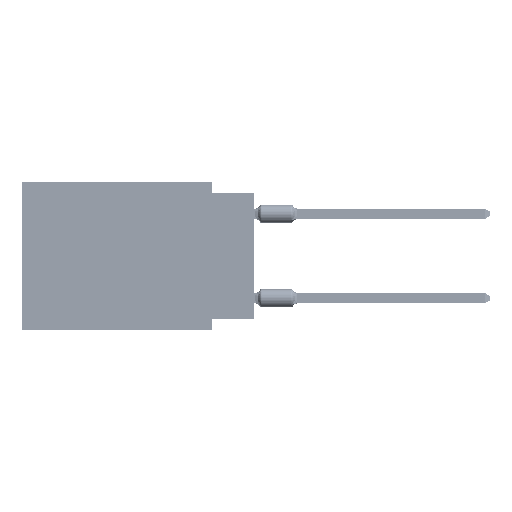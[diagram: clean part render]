
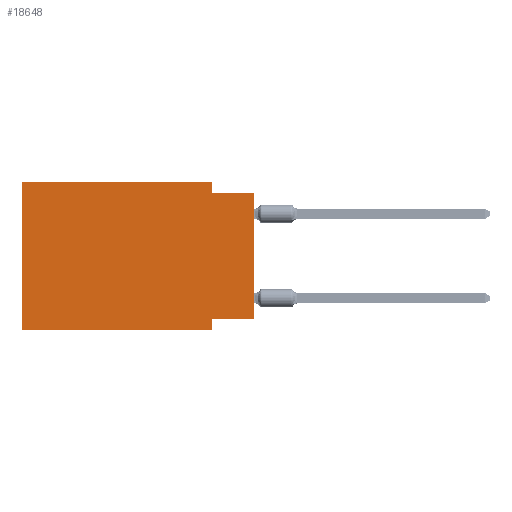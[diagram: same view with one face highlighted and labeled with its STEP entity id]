
A CAD part, left-side view. The second image highlights one B-rep face of the part: STEP entity #18648.
In plain terms, the highlighted planar face has unit normal (-1, 0, 0).
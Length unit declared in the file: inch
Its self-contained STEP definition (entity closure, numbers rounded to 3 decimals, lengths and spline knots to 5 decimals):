
#1255 = VERTEX_POINT ( 'NONE', #31636 ) ;
#1350 = EDGE_CURVE ( 'NONE', #70634, #8114, #46637, .T. ) ;
#3632 = ORIENTED_EDGE ( 'NONE', *, *, #26563, .T. ) ;
#4071 = LINE ( 'NONE', #10795, #54244 ) ;
#4739 = DIRECTION ( 'NONE',  ( 0., 0., 1. ) ) ;
#6099 = VECTOR ( 'NONE', #80054, 39.37008 ) ;
#6682 = ORIENTED_EDGE ( 'NONE', *, *, #34591, .F. ) ;
#6971 = EDGE_CURVE ( 'NONE', #55700, #53142, #4071, .T. ) ;
#7519 = EDGE_CURVE ( 'NONE', #1255, #55700, #9159, .T. ) ;
#8114 = VERTEX_POINT ( 'NONE', #39401 ) ;
#8836 = ORIENTED_EDGE ( 'NONE', *, *, #7519, .F. ) ;
#8991 = DIRECTION ( 'NONE',  ( 1., 0., 0. ) ) ;
#9159 = LINE ( 'NONE', #22427, #59217 ) ;
#9866 = DIRECTION ( 'NONE',  ( 0., 0., -1. ) ) ;
#10310 = VERTEX_POINT ( 'NONE', #69260 ) ;
#10795 = CARTESIAN_POINT ( 'NONE',  ( 0., 0., -0.025 ) ) ;
#11012 = LINE ( 'NONE', #73951, #26374 ) ;
#14127 = EDGE_CURVE ( 'NONE', #47273, #53142, #49328, .T. ) ;
#14296 = EDGE_CURVE ( 'NONE', #47273, #53185, #73774, .T. ) ;
#17582 = VECTOR ( 'NONE', #65293, 39.37008 ) ;
#18219 = CARTESIAN_POINT ( 'NONE',  ( 0., 0., 0. ) ) ;
#18648 = ADVANCED_FACE ( 'NONE', ( #41295 ), #28446, .F. ) ;
#19945 = ORIENTED_EDGE ( 'NONE', *, *, #6971, .F. ) ;
#20330 = DIRECTION ( 'NONE',  ( 0., -1., 0. ) ) ;
#21997 = CARTESIAN_POINT ( 'NONE',  ( 0., 0.55, -0.35 ) ) ;
#22427 = CARTESIAN_POINT ( 'NONE',  ( 0., 0.1, 0. ) ) ;
#24600 = EDGE_CURVE ( 'NONE', #8114, #1255, #81831, .T. ) ;
#26212 = CARTESIAN_POINT ( 'NONE',  ( 0., 0., -0.325 ) ) ;
#26374 = VECTOR ( 'NONE', #48026, 39.37008 ) ;
#26563 = EDGE_CURVE ( 'NONE', #70634, #10310, #11012, .T. ) ;
#28446 = PLANE ( 'NONE',  #42742 ) ;
#29274 = VECTOR ( 'NONE', #78388, 39.37008 ) ;
#29802 = VECTOR ( 'NONE', #20330, 39.37008 ) ;
#31636 = CARTESIAN_POINT ( 'NONE',  ( 0., 0.1, 0. ) ) ;
#32499 = EDGE_LOOP ( 'NONE', ( #65404, #19945, #8836, #62683, #41737, #3632, #6682, #44128 ) ) ;
#34020 = VECTOR ( 'NONE', #4739, 39.37008 ) ;
#34437 = CARTESIAN_POINT ( 'NONE',  ( 0., 0.1, -0.35 ) ) ;
#34591 = EDGE_CURVE ( 'NONE', #53185, #10310, #67433, .T. ) ;
#36851 = DIRECTION ( 'NONE',  ( 0., -1., 0. ) ) ;
#39401 = CARTESIAN_POINT ( 'NONE',  ( 0., 0.55, 0. ) ) ;
#41295 = FACE_OUTER_BOUND ( 'NONE', #32499, .T. ) ;
#41737 = ORIENTED_EDGE ( 'NONE', *, *, #1350, .F. ) ;
#42742 = AXIS2_PLACEMENT_3D ( 'NONE', #80630, #8991, #54689 ) ;
#44128 = ORIENTED_EDGE ( 'NONE', *, *, #14296, .F. ) ;
#46637 = LINE ( 'NONE', #84563, #29274 ) ;
#47273 = VERTEX_POINT ( 'NONE', #76887 ) ;
#48026 = DIRECTION ( 'NONE',  ( 0., -1., 0. ) ) ;
#49328 = LINE ( 'NONE', #18219, #34020 ) ;
#53142 = VERTEX_POINT ( 'NONE', #71591 ) ;
#53185 = VERTEX_POINT ( 'NONE', #72151 ) ;
#54244 = VECTOR ( 'NONE', #36851, 39.37008 ) ;
#54689 = DIRECTION ( 'NONE',  ( 0., 0., -1. ) ) ;
#55700 = VERTEX_POINT ( 'NONE', #75959 ) ;
#59217 = VECTOR ( 'NONE', #9866, 39.37008 ) ;
#62683 = ORIENTED_EDGE ( 'NONE', *, *, #24600, .F. ) ;
#65293 = DIRECTION ( 'NONE',  ( 0., 1., 0. ) ) ;
#65404 = ORIENTED_EDGE ( 'NONE', *, *, #14127, .T. ) ;
#67433 = LINE ( 'NONE', #34437, #6099 ) ;
#69260 = CARTESIAN_POINT ( 'NONE',  ( 0., 0.1, -0.35 ) ) ;
#70634 = VERTEX_POINT ( 'NONE', #21997 ) ;
#71591 = CARTESIAN_POINT ( 'NONE',  ( 0., 0., -0.025 ) ) ;
#72151 = CARTESIAN_POINT ( 'NONE',  ( 0., 0.1, -0.325 ) ) ;
#72571 = CARTESIAN_POINT ( 'NONE',  ( 0., 0.55, 0. ) ) ;
#73774 = LINE ( 'NONE', #26212, #17582 ) ;
#73951 = CARTESIAN_POINT ( 'NONE',  ( 0., 0.55, -0.35 ) ) ;
#75959 = CARTESIAN_POINT ( 'NONE',  ( 0., 0.1, -0.025 ) ) ;
#76887 = CARTESIAN_POINT ( 'NONE',  ( 0., 0., -0.325 ) ) ;
#78388 = DIRECTION ( 'NONE',  ( 0., 0., 1. ) ) ;
#80054 = DIRECTION ( 'NONE',  ( 0., 0., -1. ) ) ;
#80630 = CARTESIAN_POINT ( 'NONE',  ( 0., 0.55, 0. ) ) ;
#81831 = LINE ( 'NONE', #72571, #29802 ) ;
#84563 = CARTESIAN_POINT ( 'NONE',  ( 0., 0.55, 0. ) ) ;
